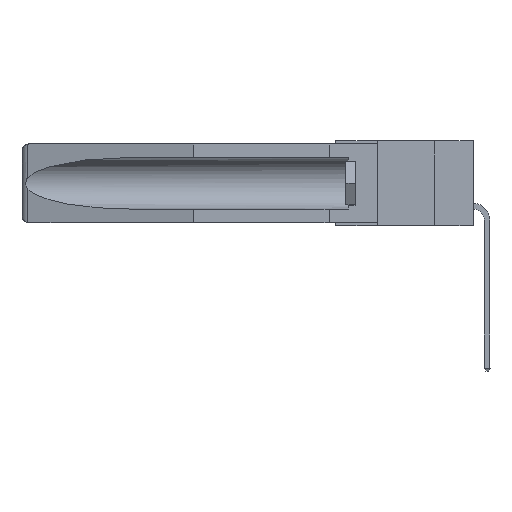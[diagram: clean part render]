
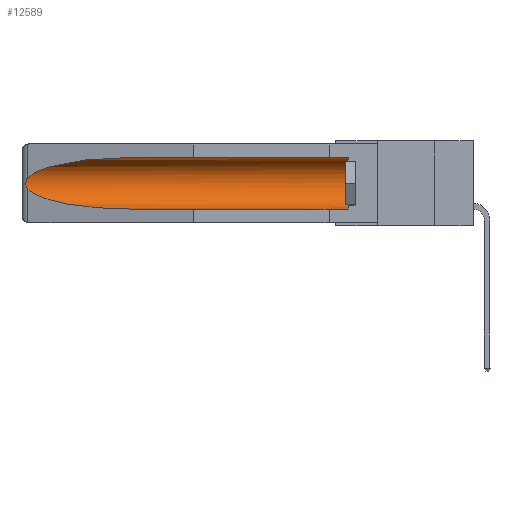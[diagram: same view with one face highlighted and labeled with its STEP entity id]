
A CAD part, left-side view. The second image highlights one B-rep face of the part: STEP entity #12589.
In plain terms, the highlighted cylindrical face has radius 2.857 mm (diameter 5.715 mm), a partial arc.
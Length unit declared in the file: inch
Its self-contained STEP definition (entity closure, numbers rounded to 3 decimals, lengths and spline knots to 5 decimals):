
#151 = VERTEX_POINT ( 'NONE', #6047 ) ;
#322 = CARTESIAN_POINT ( 'NONE',  ( 0.26597, 1.5296, -0.19026 ) ) ;
#1143 = CARTESIAN_POINT ( 'NONE',  ( 0.26597, 1.52961, -0.15275 ) ) ;
#1399 = CYLINDRICAL_SURFACE ( 'NONE', #5831, 0.1125 ) ;
#1521 = ORIENTED_EDGE ( 'NONE', *, *, #6599, .T. ) ;
#2212 = EDGE_LOOP ( 'NONE', ( #7762, #12933, #14379, #7282, #1521, #6313 ) ) ;
#2376 = CARTESIAN_POINT ( 'NONE',  ( 0.155, -0.30754, -0.284 ) ) ;
#3626 = LINE ( 'NONE', #2376, #7931 ) ;
#3833 = CARTESIAN_POINT ( 'NONE',  ( 0.2675, 1.53308, -0.17534 ) ) ;
#4093 = FACE_OUTER_BOUND ( 'NONE', #2212, .T. ) ;
#4150 = DIRECTION ( 'NONE',  ( 0., 1., 0. ) ) ;
#4556 = DIRECTION ( 'NONE',  ( 0., 1., 0. ) ) ;
#4881 = CARTESIAN_POINT ( 'NONE',  ( 0.21114, 1.30732, -0.059 ) ) ;
#4947 =( BOUNDED_CURVE ( )  B_SPLINE_CURVE ( 3, ( #14022, #11447, #13904, #12757 ),
 .UNSPECIFIED., .F., .F. ) 
 B_SPLINE_CURVE_WITH_KNOTS ( ( 4, 4 ),
 ( 0.1948, 1.5708 ),
 .UNSPECIFIED. ) 
 CURVE ( )  GEOMETRIC_REPRESENTATION_ITEM ( )  RATIONAL_B_SPLINE_CURVE ( ( 1., 0.848, 0.848, 1. ) ) 
 REPRESENTATION_ITEM ( '' )  );
#5106 = VERTEX_POINT ( 'NONE', #14324 ) ;
#5195 = EDGE_CURVE ( 'NONE', #7921, #12459, #15553, .T. ) ;
#5274 = CARTESIAN_POINT ( 'NONE',  ( 0.2673, 1.5327, -0.16383 ) ) ;
#5831 = AXIS2_PLACEMENT_3D ( 'NONE', #8411, #4556, #6957 ) ;
#6013 = VECTOR ( 'NONE', #4150, 39.37008 ) ;
#6047 = CARTESIAN_POINT ( 'NONE',  ( 0.155, 0.126, -0.284 ) ) ;
#6152 = DIRECTION ( 'NONE',  ( 0., 1., 0. ) ) ;
#6313 = ORIENTED_EDGE ( 'NONE', *, *, #5195, .T. ) ;
#6558 = CARTESIAN_POINT ( 'NONE',  ( 0.155, -0.30754, -0.059 ) ) ;
#6599 = EDGE_CURVE ( 'NONE', #151, #7921, #12380, .T. ) ;
#6902 = EDGE_CURVE ( 'NONE', #151, #13455, #3626, .T. ) ;
#6957 = DIRECTION ( 'NONE',  ( 0., 0., 1. ) ) ;
#7264 = AXIS2_PLACEMENT_3D ( 'NONE', #10194, #10242, #11394 ) ;
#7282 = ORIENTED_EDGE ( 'NONE', *, *, #6902, .F. ) ;
#7762 = ORIENTED_EDGE ( 'NONE', *, *, #8091, .T. ) ;
#7921 = VERTEX_POINT ( 'NONE', #14286 ) ;
#7931 = VECTOR ( 'NONE', #6152, 39.37008 ) ;
#8084 = CARTESIAN_POINT ( 'NONE',  ( 0.26537, 1.52718, -0.14972 ) ) ;
#8091 = EDGE_CURVE ( 'NONE', #12459, #5106, #9835, .T. ) ;
#8411 = CARTESIAN_POINT ( 'NONE',  ( 0.155, -0.30754, -0.1715 ) ) ;
#8412 = EDGE_CURVE ( 'NONE', #5106, #9972, #10982, .T. ) ;
#9033 = CARTESIAN_POINT ( 'NONE',  ( 0.26537, 1.52718, -0.19328 ) ) ;
#9835 =( BOUNDED_CURVE ( )  B_SPLINE_CURVE ( 3, ( #12458, #4881, #11309, #8084 ),
 .UNSPECIFIED., .F., .F. ) 
 B_SPLINE_CURVE_WITH_KNOTS ( ( 4, 4 ),
 ( 4.71239, 6.08839 ),
 .UNSPECIFIED. ) 
 CURVE ( )  GEOMETRIC_REPRESENTATION_ITEM ( )  RATIONAL_B_SPLINE_CURVE ( ( 1., 0.848, 0.848, 1. ) ) 
 REPRESENTATION_ITEM ( '' )  );
#9972 = VERTEX_POINT ( 'NONE', #13835 ) ;
#10194 = CARTESIAN_POINT ( 'NONE',  ( 0.155, 0.126, -0.1715 ) ) ;
#10242 = DIRECTION ( 'NONE',  ( 0., -1., 0. ) ) ;
#10447 = EDGE_CURVE ( 'NONE', #9972, #13455, #4947, .T. ) ;
#10982 = B_SPLINE_CURVE_WITH_KNOTS ( 'NONE', 3,
 ( #11370, #1143, #11041, #5274, #13932, #3833, #12518, #15040, #322, #9033 ),
 .UNSPECIFIED., .F., .F.,
 ( 4, 2, 2, 2, 4 ),
 ( 0., 0.00029, 0.00058, 0.00087, 0.00117 ),
 .UNSPECIFIED. ) ;
#11041 = CARTESIAN_POINT ( 'NONE',  ( 0.26654, 1.53092, -0.15636 ) ) ;
#11309 = CARTESIAN_POINT ( 'NONE',  ( 0.25451, 1.48313, -0.09465 ) ) ;
#11370 = CARTESIAN_POINT ( 'NONE',  ( 0.26537, 1.52718, -0.14972 ) ) ;
#11394 = DIRECTION ( 'NONE',  ( 0., 0., 1. ) ) ;
#11447 = CARTESIAN_POINT ( 'NONE',  ( 0.25451, 1.48313, -0.24835 ) ) ;
#12380 = CIRCLE ( 'NONE', #7264, 0.1125 ) ;
#12458 = CARTESIAN_POINT ( 'NONE',  ( 0.155, 1.07973, -0.059 ) ) ;
#12459 = VERTEX_POINT ( 'NONE', #15870 ) ;
#12518 = CARTESIAN_POINT ( 'NONE',  ( 0.2673, 1.53269, -0.17917 ) ) ;
#12589 = ADVANCED_FACE ( 'NONE', ( #4093 ), #1399, .F. ) ;
#12757 = CARTESIAN_POINT ( 'NONE',  ( 0.155, 1.07973, -0.284 ) ) ;
#12933 = ORIENTED_EDGE ( 'NONE', *, *, #8412, .T. ) ;
#13384 = CARTESIAN_POINT ( 'NONE',  ( 0.155, 1.07973, -0.284 ) ) ;
#13455 = VERTEX_POINT ( 'NONE', #13384 ) ;
#13835 = CARTESIAN_POINT ( 'NONE',  ( 0.26537, 1.52718, -0.19328 ) ) ;
#13904 = CARTESIAN_POINT ( 'NONE',  ( 0.21114, 1.30732, -0.284 ) ) ;
#13932 = CARTESIAN_POINT ( 'NONE',  ( 0.2675, 1.53308, -0.16763 ) ) ;
#14022 = CARTESIAN_POINT ( 'NONE',  ( 0.26537, 1.52718, -0.19328 ) ) ;
#14286 = CARTESIAN_POINT ( 'NONE',  ( 0.155, 0.126, -0.059 ) ) ;
#14324 = CARTESIAN_POINT ( 'NONE',  ( 0.26537, 1.52718, -0.14972 ) ) ;
#14379 = ORIENTED_EDGE ( 'NONE', *, *, #10447, .T. ) ;
#15040 = CARTESIAN_POINT ( 'NONE',  ( 0.26655, 1.53094, -0.18657 ) ) ;
#15553 = LINE ( 'NONE', #6558, #6013 ) ;
#15870 = CARTESIAN_POINT ( 'NONE',  ( 0.155, 1.07973, -0.059 ) ) ;
